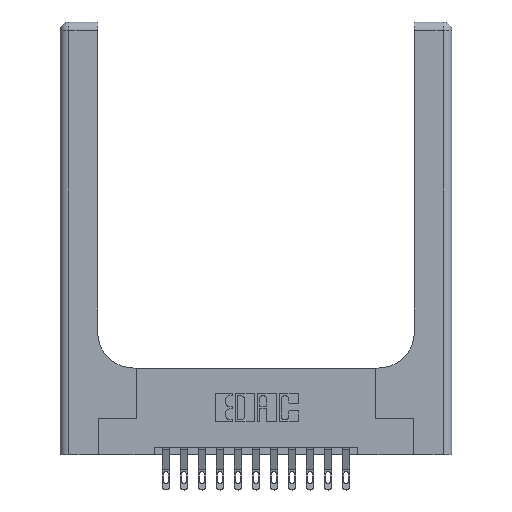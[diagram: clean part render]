
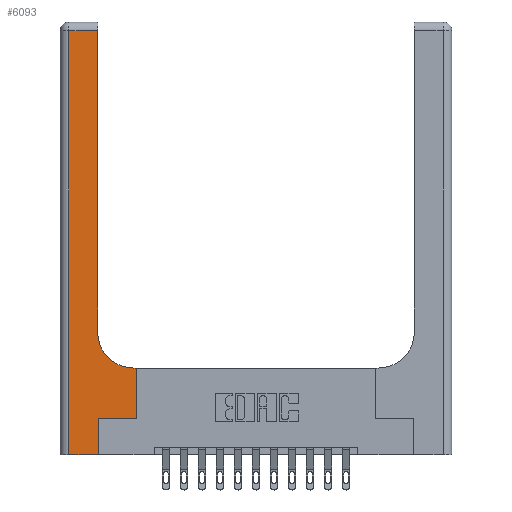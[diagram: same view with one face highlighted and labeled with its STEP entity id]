
A CAD part, top view. The second image highlights one B-rep face of the part: STEP entity #6093.
In plain terms, the highlighted planar face has unit normal (0, 0, 1).
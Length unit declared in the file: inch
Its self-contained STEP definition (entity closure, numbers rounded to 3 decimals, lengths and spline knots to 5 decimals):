
#274 = CARTESIAN_POINT ( 'NONE',  ( 0.06, 3., 0.37 ) ) ;
#870 = CARTESIAN_POINT ( 'NONE',  ( 0.06, 2.94, 0.37 ) ) ;
#1159 = VECTOR ( 'NONE', #11007, 39.37008 ) ;
#1454 = DIRECTION ( 'NONE',  ( 1., 0., 0. ) ) ;
#1466 = LINE ( 'NONE', #12326, #1159 ) ;
#2380 = CARTESIAN_POINT ( 'NONE',  ( 0., 2.94, 0.37 ) ) ;
#2722 = VERTEX_POINT ( 'NONE', #12979 ) ;
#3120 = VECTOR ( 'NONE', #11846, 39.37008 ) ;
#3326 = EDGE_LOOP ( 'NONE', ( #4587, #13322, #14100, #11044, #4052, #10354, #10616, #16947, #5296 ) ) ;
#3457 = LINE ( 'NONE', #12898, #14860 ) ;
#3490 = PLANE ( 'NONE',  #6300 ) ;
#3539 = CARTESIAN_POINT ( 'NONE',  ( 0.51, 0.85, 0.37 ) ) ;
#3552 = VERTEX_POINT ( 'NONE', #14342 ) ;
#3923 = VERTEX_POINT ( 'NONE', #10551 ) ;
#4052 = ORIENTED_EDGE ( 'NONE', *, *, #8077, .T. ) ;
#4193 = EDGE_CURVE ( 'NONE', #10480, #9161, #10610, .T. ) ;
#4252 = CIRCLE ( 'NONE', #10356, 0.25 ) ;
#4273 = CARTESIAN_POINT ( 'NONE',  ( 0.26, 2.94, 0.37 ) ) ;
#4587 = ORIENTED_EDGE ( 'NONE', *, *, #4193, .T. ) ;
#4922 = CARTESIAN_POINT ( 'NONE',  ( 0.06, 0., 0.37 ) ) ;
#5296 = ORIENTED_EDGE ( 'NONE', *, *, #15023, .T. ) ;
#5629 = DIRECTION ( 'NONE',  ( 0., -1., 0. ) ) ;
#5694 = VECTOR ( 'NONE', #6475, 39.37008 ) ;
#5853 = CARTESIAN_POINT ( 'NONE',  ( 0.265, 0.25, 0.37 ) ) ;
#6063 = CARTESIAN_POINT ( 'NONE',  ( 0.528, 0.6, 0.37 ) ) ;
#6093 = ADVANCED_FACE ( 'NONE', ( #15324 ), #3490, .F. ) ;
#6164 = CARTESIAN_POINT ( 'NONE',  ( 0., 3., 0.37 ) ) ;
#6300 = AXIS2_PLACEMENT_3D ( 'NONE', #6164, #14079, #16888 ) ;
#6393 = DIRECTION ( 'NONE',  ( 0., 0., -1. ) ) ;
#6475 = DIRECTION ( 'NONE',  ( -1., 0., 0. ) ) ;
#7044 = VECTOR ( 'NONE', #5629, 39.37008 ) ;
#7618 = DIRECTION ( 'NONE',  ( 1., 0., 0. ) ) ;
#8077 = EDGE_CURVE ( 'NONE', #3552, #3923, #12614, .T. ) ;
#8208 = VECTOR ( 'NONE', #1454, 39.37008 ) ;
#8926 = VERTEX_POINT ( 'NONE', #4922 ) ;
#9161 = VERTEX_POINT ( 'NONE', #4273 ) ;
#9184 = EDGE_CURVE ( 'NONE', #16282, #8926, #15103, .T. ) ;
#9852 = VECTOR ( 'NONE', #7618, 39.37008 ) ;
#10316 = EDGE_CURVE ( 'NONE', #15777, #2722, #3457, .T. ) ;
#10354 = ORIENTED_EDGE ( 'NONE', *, *, #12391, .T. ) ;
#10356 = AXIS2_PLACEMENT_3D ( 'NONE', #3539, #6393, #15542 ) ;
#10480 = VERTEX_POINT ( 'NONE', #14918 ) ;
#10551 = CARTESIAN_POINT ( 'NONE',  ( 0.265, 0.25, 0.37 ) ) ;
#10610 = LINE ( 'NONE', #16000, #3120 ) ;
#10616 = ORIENTED_EDGE ( 'NONE', *, *, #12936, .T. ) ;
#11007 = DIRECTION ( 'NONE',  ( 0., 1., 0. ) ) ;
#11044 = ORIENTED_EDGE ( 'NONE', *, *, #13289, .T. ) ;
#11565 = DIRECTION ( 'NONE',  ( -1., 0., 0. ) ) ;
#11846 = DIRECTION ( 'NONE',  ( 0., 1., 0. ) ) ;
#12238 = CARTESIAN_POINT ( 'NONE',  ( 0.265, 0., 0.37 ) ) ;
#12326 = CARTESIAN_POINT ( 'NONE',  ( 0.528, 0.25, 0.37 ) ) ;
#12342 = DIRECTION ( 'NONE',  ( 0., 1., 0. ) ) ;
#12391 = EDGE_CURVE ( 'NONE', #3923, #15954, #13477, .T. ) ;
#12614 = LINE ( 'NONE', #12238, #16498 ) ;
#12898 = CARTESIAN_POINT ( 'NONE',  ( 0.26, 0.6, 0.37 ) ) ;
#12936 = EDGE_CURVE ( 'NONE', #15954, #15777, #1466, .T. ) ;
#12979 = CARTESIAN_POINT ( 'NONE',  ( 0.51, 0.6, 0.37 ) ) ;
#13129 = CARTESIAN_POINT ( 'NONE',  ( 0.528, 0.25, 0.37 ) ) ;
#13289 = EDGE_CURVE ( 'NONE', #8926, #3552, #17215, .T. ) ;
#13295 = CARTESIAN_POINT ( 'NONE',  ( 0., 0., 0.37 ) ) ;
#13322 = ORIENTED_EDGE ( 'NONE', *, *, #15099, .T. ) ;
#13477 = LINE ( 'NONE', #5853, #8208 ) ;
#14079 = DIRECTION ( 'NONE',  ( 0., 0., -1. ) ) ;
#14100 = ORIENTED_EDGE ( 'NONE', *, *, #9184, .T. ) ;
#14342 = CARTESIAN_POINT ( 'NONE',  ( 0.265, 0., 0.37 ) ) ;
#14558 = LINE ( 'NONE', #2380, #5694 ) ;
#14860 = VECTOR ( 'NONE', #11565, 39.37008 ) ;
#14918 = CARTESIAN_POINT ( 'NONE',  ( 0.26, 0.85, 0.37 ) ) ;
#15023 = EDGE_CURVE ( 'NONE', #2722, #10480, #4252, .T. ) ;
#15099 = EDGE_CURVE ( 'NONE', #9161, #16282, #14558, .T. ) ;
#15103 = LINE ( 'NONE', #274, #7044 ) ;
#15324 = FACE_OUTER_BOUND ( 'NONE', #3326, .T. ) ;
#15542 = DIRECTION ( 'NONE',  ( 1., 0., 0. ) ) ;
#15777 = VERTEX_POINT ( 'NONE', #6063 ) ;
#15954 = VERTEX_POINT ( 'NONE', #13129 ) ;
#16000 = CARTESIAN_POINT ( 'NONE',  ( 0.26, 3., 0.37 ) ) ;
#16282 = VERTEX_POINT ( 'NONE', #870 ) ;
#16498 = VECTOR ( 'NONE', #12342, 39.37008 ) ;
#16888 = DIRECTION ( 'NONE',  ( -1., 0., 0. ) ) ;
#16947 = ORIENTED_EDGE ( 'NONE', *, *, #10316, .T. ) ;
#17215 = LINE ( 'NONE', #13295, #9852 ) ;
